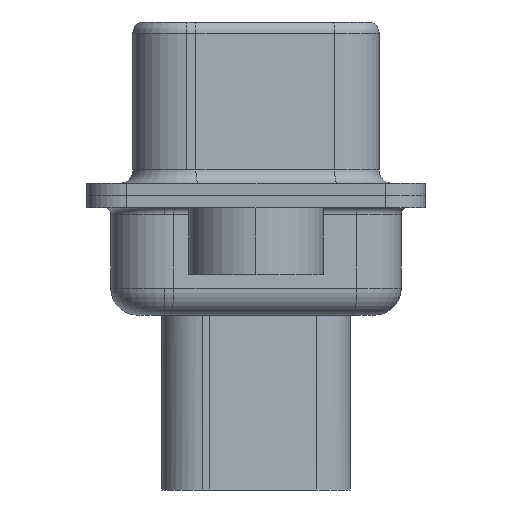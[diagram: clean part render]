
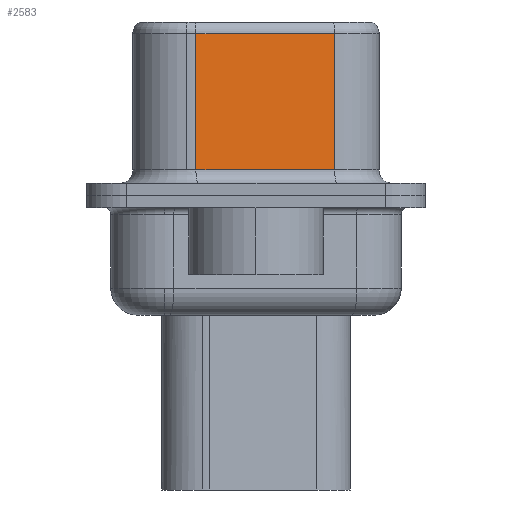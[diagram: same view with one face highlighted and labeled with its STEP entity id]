
A CAD part, left-side view. The second image highlights one B-rep face of the part: STEP entity #2583.
In plain terms, the highlighted planar face has unit normal (-0.985, -0.174, 0).
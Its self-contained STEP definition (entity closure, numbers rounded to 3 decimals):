
#206 = LINE ( 'NONE', #17004, #16619 ) ;
#553 = VECTOR ( 'NONE', #8583, 1000. ) ;
#1181 = EDGE_CURVE ( 'NONE', #12652, #15886, #2242, .T. ) ;
#1342 = ORIENTED_EDGE ( 'NONE', *, *, #17707, .T. ) ;
#2143 = CARTESIAN_POINT ( 'NONE',  ( 3.67, 2.233, 6.02 ) ) ;
#2242 = LINE ( 'NONE', #13268, #5190 ) ;
#2477 = ORIENTED_EDGE ( 'NONE', *, *, #7828, .T. ) ;
#2583 = ADVANCED_FACE ( 'NONE', ( #18034 ), #10784, .F. ) ;
#2781 = VERTEX_POINT ( 'NONE', #3577 ) ;
#2791 = LINE ( 'NONE', #11244, #553 ) ;
#3350 = CARTESIAN_POINT ( 'NONE',  ( 4.58, -2.927, 0.95 ) ) ;
#3577 = CARTESIAN_POINT ( 'NONE',  ( 4.58, -2.927, 6.02 ) ) ;
#3625 = DIRECTION ( 'NONE',  ( -0.174, 0.985, 0. ) ) ;
#5190 = VECTOR ( 'NONE', #9238, 1000. ) ;
#6514 = EDGE_CURVE ( 'NONE', #2781, #14045, #206, .T. ) ;
#7067 = ORIENTED_EDGE ( 'NONE', *, *, #1181, .T. ) ;
#7399 = ORIENTED_EDGE ( 'NONE', *, *, #6514, .F. ) ;
#7828 = EDGE_CURVE ( 'NONE', #2781, #12652, #2791, .T. ) ;
#8583 = DIRECTION ( 'NONE',  ( -0.174, 0.985, 0. ) ) ;
#8888 = CARTESIAN_POINT ( 'NONE',  ( 3.67, 2.233, 0.95 ) ) ;
#9238 = DIRECTION ( 'NONE',  ( 0., 0., -1. ) ) ;
#9419 = CARTESIAN_POINT ( 'NONE',  ( 4.58, -2.927, 6.52 ) ) ;
#9867 = DIRECTION ( 'NONE',  ( 0., 0., -1. ) ) ;
#10604 = DIRECTION ( 'NONE',  ( 0.985, 0.174, 0. ) ) ;
#10784 = PLANE ( 'NONE',  #15904 ) ;
#11244 = CARTESIAN_POINT ( 'NONE',  ( 4.58, -2.927, 6.02 ) ) ;
#11577 = VECTOR ( 'NONE', #17286, 1000. ) ;
#11786 = LINE ( 'NONE', #15909, #11577 ) ;
#12652 = VERTEX_POINT ( 'NONE', #2143 ) ;
#13268 = CARTESIAN_POINT ( 'NONE',  ( 3.67, 2.233, 6.52 ) ) ;
#14045 = VERTEX_POINT ( 'NONE', #3350 ) ;
#15886 = VERTEX_POINT ( 'NONE', #8888 ) ;
#15904 = AXIS2_PLACEMENT_3D ( 'NONE', #9419, #10604, #3625 ) ;
#15909 = CARTESIAN_POINT ( 'NONE',  ( 4.58, -2.927, 0.95 ) ) ;
#16060 = EDGE_LOOP ( 'NONE', ( #7399, #2477, #7067, #1342 ) ) ;
#16619 = VECTOR ( 'NONE', #9867, 1000. ) ;
#17004 = CARTESIAN_POINT ( 'NONE',  ( 4.58, -2.927, 6.52 ) ) ;
#17286 = DIRECTION ( 'NONE',  ( 0.174, -0.985, 0. ) ) ;
#17707 = EDGE_CURVE ( 'NONE', #15886, #14045, #11786, .T. ) ;
#18034 = FACE_OUTER_BOUND ( 'NONE', #16060, .T. ) ;
